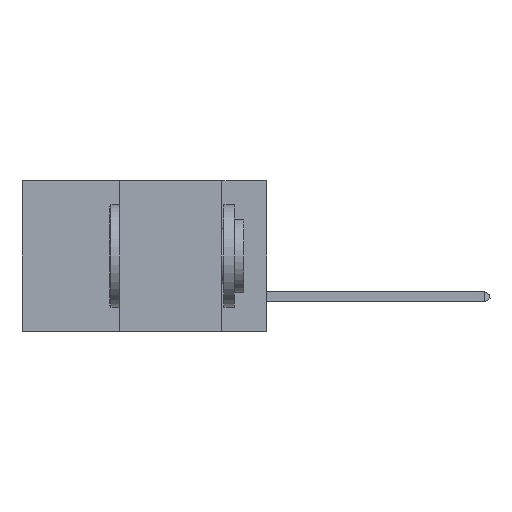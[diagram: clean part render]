
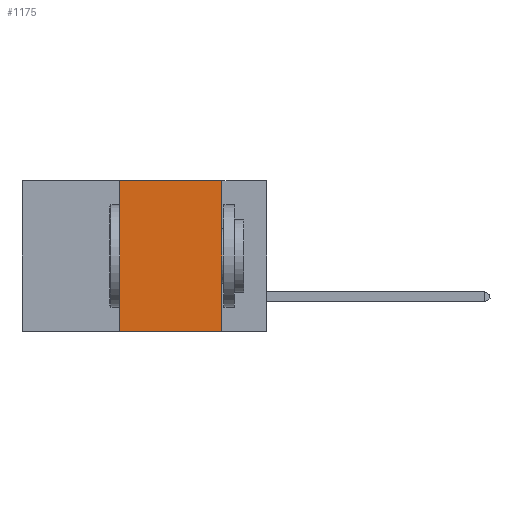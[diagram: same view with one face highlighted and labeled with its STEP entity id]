
A CAD part, left-side view. The second image highlights one B-rep face of the part: STEP entity #1175.
In plain terms, the highlighted planar face has unit normal (-1, 0, 0).
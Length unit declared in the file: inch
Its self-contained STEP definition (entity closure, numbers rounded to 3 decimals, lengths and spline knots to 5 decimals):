
#436 = CARTESIAN_POINT ( 'NONE',  ( 0., 0.11, 0. ) ) ;
#482 = FACE_OUTER_BOUND ( 'NONE', #8065, .T. ) ;
#781 = DIRECTION ( 'NONE',  ( 0., 0., -1. ) ) ;
#946 = VERTEX_POINT ( 'NONE', #11728 ) ;
#1175 = ADVANCED_FACE ( 'NONE', ( #482 ), #5874, .F. ) ;
#1359 = AXIS2_PLACEMENT_3D ( 'NONE', #5976, #5848, #5829 ) ;
#2194 = DIRECTION ( 'NONE',  ( 0., 0., 1. ) ) ;
#2197 = EDGE_CURVE ( 'NONE', #946, #7440, #12524, .T. ) ;
#2422 = LINE ( 'NONE', #9835, #2746 ) ;
#2439 = CARTESIAN_POINT ( 'NONE',  ( 0., 0.36, 0. ) ) ;
#2525 = LINE ( 'NONE', #11037, #7613 ) ;
#2746 = VECTOR ( 'NONE', #9794, 39.37008 ) ;
#3203 = DIRECTION ( 'NONE',  ( 0., -1., 0. ) ) ;
#3608 = ORIENTED_EDGE ( 'NONE', *, *, #6999, .F. ) ;
#4276 = CARTESIAN_POINT ( 'NONE',  ( 0., 0.11, -0.37 ) ) ;
#5829 = DIRECTION ( 'NONE',  ( 0., 0., -1. ) ) ;
#5848 = DIRECTION ( 'NONE',  ( 1., 0., 0. ) ) ;
#5874 = PLANE ( 'NONE',  #1359 ) ;
#5976 = CARTESIAN_POINT ( 'NONE',  ( 0., 0.6, 0. ) ) ;
#6292 = VERTEX_POINT ( 'NONE', #6612 ) ;
#6459 = VERTEX_POINT ( 'NONE', #4276 ) ;
#6612 = CARTESIAN_POINT ( 'NONE',  ( 0., 0.11, 0. ) ) ;
#6633 = ORIENTED_EDGE ( 'NONE', *, *, #2197, .F. ) ;
#6999 = EDGE_CURVE ( 'NONE', #6292, #6459, #8120, .T. ) ;
#7151 = CARTESIAN_POINT ( 'NONE',  ( 0., 0.36, 0. ) ) ;
#7303 = VECTOR ( 'NONE', #2194, 39.37008 ) ;
#7440 = VERTEX_POINT ( 'NONE', #7151 ) ;
#7613 = VECTOR ( 'NONE', #3203, 39.37008 ) ;
#8065 = EDGE_LOOP ( 'NONE', ( #3608, #11371, #6633, #9229 ) ) ;
#8120 = LINE ( 'NONE', #436, #8409 ) ;
#8409 = VECTOR ( 'NONE', #781, 39.37008 ) ;
#9178 = EDGE_CURVE ( 'NONE', #946, #6459, #2422, .T. ) ;
#9229 = ORIENTED_EDGE ( 'NONE', *, *, #9178, .T. ) ;
#9794 = DIRECTION ( 'NONE',  ( 0., -1., 0. ) ) ;
#9835 = CARTESIAN_POINT ( 'NONE',  ( 0., 0.6, -0.37 ) ) ;
#11037 = CARTESIAN_POINT ( 'NONE',  ( 0., 0.6, 0. ) ) ;
#11371 = ORIENTED_EDGE ( 'NONE', *, *, #11639, .F. ) ;
#11639 = EDGE_CURVE ( 'NONE', #7440, #6292, #2525, .T. ) ;
#11728 = CARTESIAN_POINT ( 'NONE',  ( 0., 0.36, -0.37 ) ) ;
#12524 = LINE ( 'NONE', #2439, #7303 ) ;
